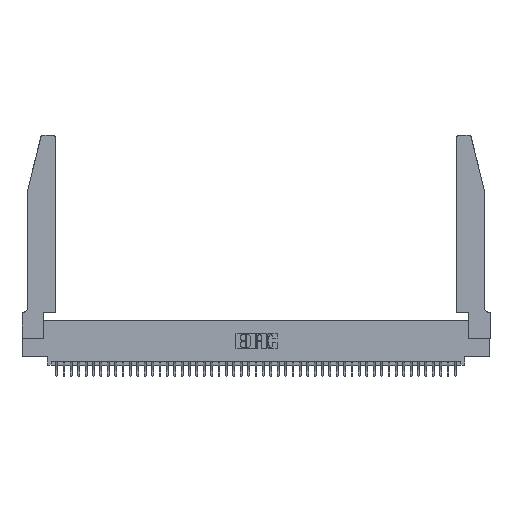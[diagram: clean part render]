
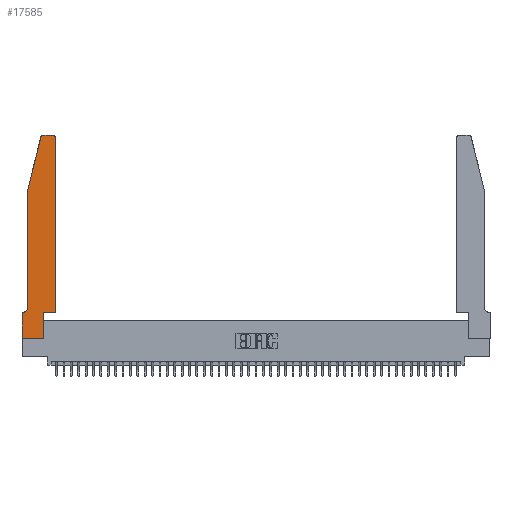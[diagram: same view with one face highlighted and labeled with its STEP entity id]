
A CAD part, top view. The second image highlights one B-rep face of the part: STEP entity #17585.
In plain terms, the highlighted planar face has unit normal (0, 0, 1).
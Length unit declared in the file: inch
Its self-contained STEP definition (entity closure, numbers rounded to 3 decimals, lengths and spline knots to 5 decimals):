
#538 = VECTOR ( 'NONE', #25770, 39.37008 ) ;
#815 = CIRCLE ( 'NONE', #19973, 0.07 ) ;
#1586 = EDGE_CURVE ( 'NONE', #19823, #18015, #17765, .T. ) ;
#2726 = VECTOR ( 'NONE', #23477, 39.37008 ) ;
#3754 = VERTEX_POINT ( 'NONE', #32100 ) ;
#3792 = ORIENTED_EDGE ( 'NONE', *, *, #26870, .T. ) ;
#3825 = AXIS2_PLACEMENT_3D ( 'NONE', #6704, #35289, #6082 ) ;
#4029 = CARTESIAN_POINT ( 'NONE',  ( 0.0755, 2., 0.37 ) ) ;
#4063 = VECTOR ( 'NONE', #32357, 39.37008 ) ;
#4172 = EDGE_CURVE ( 'NONE', #41284, #14350, #6353, .T. ) ;
#4333 = LINE ( 'NONE', #42284, #36367 ) ;
#5212 = AXIS2_PLACEMENT_3D ( 'NONE', #14650, #7881, #11358 ) ;
#6032 = CARTESIAN_POINT ( 'NONE',  ( 0., 0., 0.37 ) ) ;
#6082 = DIRECTION ( 'NONE',  ( 1., 0., 0. ) ) ;
#6353 = LINE ( 'NONE', #34420, #20926 ) ;
#6704 = CARTESIAN_POINT ( 'NONE',  ( 0.4205, 2.72, 0.37 ) ) ;
#7785 = VECTOR ( 'NONE', #24430, 39.37008 ) ;
#7791 = DIRECTION ( 'NONE',  ( -0.239, -0.971, 0. ) ) ;
#7881 = DIRECTION ( 'NONE',  ( 0., 0., 1. ) ) ;
#8245 = DIRECTION ( 'NONE',  ( 0., 0., -1. ) ) ;
#8811 = CARTESIAN_POINT ( 'NONE',  ( 0.2865, 0., 0.37 ) ) ;
#9122 = LINE ( 'NONE', #39452, #4063 ) ;
#11031 = PLANE ( 'NONE',  #5212 ) ;
#11358 = DIRECTION ( 'NONE',  ( 1., 0., 0. ) ) ;
#11810 = ORIENTED_EDGE ( 'NONE', *, *, #4172, .T. ) ;
#12023 = ORIENTED_EDGE ( 'NONE', *, *, #22023, .T. ) ;
#12672 = DIRECTION ( 'NONE',  ( 0., 0., 1. ) ) ;
#13801 = ORIENTED_EDGE ( 'NONE', *, *, #44487, .T. ) ;
#14350 = VERTEX_POINT ( 'NONE', #18992 ) ;
#14650 = CARTESIAN_POINT ( 'NONE',  ( 0., 0.35, 0.37 ) ) ;
#15573 = CARTESIAN_POINT ( 'NONE',  ( 0.4505, 0.35, 0.37 ) ) ;
#15829 = EDGE_LOOP ( 'NONE', ( #20323, #28314, #13801, #29531, #16729, #11810, #28741, #21027, #28613, #3792, #32587, #12023 ) ) ;
#15952 = CARTESIAN_POINT ( 'NONE',  ( 0.4505, 0.35, 0.37 ) ) ;
#16729 = ORIENTED_EDGE ( 'NONE', *, *, #18944, .T. ) ;
#16862 = CIRCLE ( 'NONE', #3825, 0.03 ) ;
#17291 = CARTESIAN_POINT ( 'NONE',  ( 0.25487, 2.72718, 0.37 ) ) ;
#17585 = ADVANCED_FACE ( 'NONE', ( #38075 ), #11031, .T. ) ;
#17765 = CIRCLE ( 'NONE', #27639, 0.03 ) ;
#18015 = VERTEX_POINT ( 'NONE', #17291 ) ;
#18274 = CARTESIAN_POINT ( 'NONE',  ( 0., 0., 0.37 ) ) ;
#18944 = EDGE_CURVE ( 'NONE', #3754, #41284, #815, .T. ) ;
#18992 = CARTESIAN_POINT ( 'NONE',  ( 0., 0.35, 0.37 ) ) ;
#19054 = DIRECTION ( 'NONE',  ( -1., 0., 0. ) ) ;
#19436 = CARTESIAN_POINT ( 'NONE',  ( 0.0055, 0.35, 0.37 ) ) ;
#19531 = DIRECTION ( 'NONE',  ( 1., 0., 0. ) ) ;
#19630 = VERTEX_POINT ( 'NONE', #8811 ) ;
#19657 = CARTESIAN_POINT ( 'NONE',  ( 0.2865, 0.35, 0.37 ) ) ;
#19823 = VERTEX_POINT ( 'NONE', #23278 ) ;
#19973 = AXIS2_PLACEMENT_3D ( 'NONE', #22684, #8245, #19054 ) ;
#20323 = ORIENTED_EDGE ( 'NONE', *, *, #27969, .T. ) ;
#20500 = CARTESIAN_POINT ( 'NONE',  ( 0.4505, 2.72, 0.37 ) ) ;
#20820 = CARTESIAN_POINT ( 'NONE',  ( 0.2605, 2.75, 0.37 ) ) ;
#20921 = DIRECTION ( 'NONE',  ( 1., 0., 0. ) ) ;
#20926 = VECTOR ( 'NONE', #25094, 39.37008 ) ;
#21027 = ORIENTED_EDGE ( 'NONE', *, *, #28450, .T. ) ;
#21094 = EDGE_CURVE ( 'NONE', #35872, #3754, #43291, .T. ) ;
#21793 = LINE ( 'NONE', #19657, #2726 ) ;
#22023 = EDGE_CURVE ( 'NONE', #27707, #37487, #16862, .T. ) ;
#22375 = VECTOR ( 'NONE', #20921, 39.37008 ) ;
#22684 = CARTESIAN_POINT ( 'NONE',  ( 0.0055, 0.42, 0.37 ) ) ;
#23278 = CARTESIAN_POINT ( 'NONE',  ( 0.284, 2.75, 0.37 ) ) ;
#23477 = DIRECTION ( 'NONE',  ( 0., 1., 0. ) ) ;
#24430 = DIRECTION ( 'NONE',  ( -1., 0., 0. ) ) ;
#25094 = DIRECTION ( 'NONE',  ( -1., 0., 0. ) ) ;
#25174 = CARTESIAN_POINT ( 'NONE',  ( 0.0755, 2., 0.37 ) ) ;
#25770 = DIRECTION ( 'NONE',  ( 0., -1., 0. ) ) ;
#26344 = LINE ( 'NONE', #20820, #7785 ) ;
#26870 = EDGE_CURVE ( 'NONE', #32142, #33452, #44471, .T. ) ;
#27639 = AXIS2_PLACEMENT_3D ( 'NONE', #30398, #12672, #19531 ) ;
#27707 = VERTEX_POINT ( 'NONE', #20500 ) ;
#27968 = DIRECTION ( 'NONE',  ( 0., 1., 0. ) ) ;
#27969 = EDGE_CURVE ( 'NONE', #37487, #19823, #26344, .T. ) ;
#28314 = ORIENTED_EDGE ( 'NONE', *, *, #1586, .T. ) ;
#28450 = EDGE_CURVE ( 'NONE', #32233, #19630, #38135, .T. ) ;
#28613 = ORIENTED_EDGE ( 'NONE', *, *, #38099, .T. ) ;
#28741 = ORIENTED_EDGE ( 'NONE', *, *, #34393, .T. ) ;
#29072 = LINE ( 'NONE', #4029, #35833 ) ;
#29531 = ORIENTED_EDGE ( 'NONE', *, *, #21094, .T. ) ;
#29675 = CARTESIAN_POINT ( 'NONE',  ( 0.0755, 2., 0.37 ) ) ;
#30398 = CARTESIAN_POINT ( 'NONE',  ( 0.284, 2.72, 0.37 ) ) ;
#31551 = EDGE_CURVE ( 'NONE', #33452, #27707, #4333, .T. ) ;
#32100 = CARTESIAN_POINT ( 'NONE',  ( 0.0755, 0.42, 0.37 ) ) ;
#32142 = VERTEX_POINT ( 'NONE', #32897 ) ;
#32233 = VERTEX_POINT ( 'NONE', #18274 ) ;
#32357 = DIRECTION ( 'NONE',  ( 0., -1., 0. ) ) ;
#32587 = ORIENTED_EDGE ( 'NONE', *, *, #31551, .T. ) ;
#32897 = CARTESIAN_POINT ( 'NONE',  ( 0.2865, 0.35, 0.37 ) ) ;
#33452 = VERTEX_POINT ( 'NONE', #15952 ) ;
#34393 = EDGE_CURVE ( 'NONE', #14350, #32233, #9122, .T. ) ;
#34420 = CARTESIAN_POINT ( 'NONE',  ( 0.0755, 0.35, 0.37 ) ) ;
#35289 = DIRECTION ( 'NONE',  ( 0., 0., 1. ) ) ;
#35833 = VECTOR ( 'NONE', #7791, 39.37008 ) ;
#35872 = VERTEX_POINT ( 'NONE', #25174 ) ;
#36367 = VECTOR ( 'NONE', #27968, 39.37008 ) ;
#37487 = VERTEX_POINT ( 'NONE', #45820 ) ;
#38075 = FACE_OUTER_BOUND ( 'NONE', #15829, .T. ) ;
#38099 = EDGE_CURVE ( 'NONE', #19630, #32142, #21793, .T. ) ;
#38135 = LINE ( 'NONE', #6032, #22375 ) ;
#39452 = CARTESIAN_POINT ( 'NONE',  ( 0., 0., 0.37 ) ) ;
#41284 = VERTEX_POINT ( 'NONE', #19436 ) ;
#42284 = CARTESIAN_POINT ( 'NONE',  ( 0.4505, 0.35, 0.37 ) ) ;
#43291 = LINE ( 'NONE', #29675, #538 ) ;
#43327 = VECTOR ( 'NONE', #44467, 39.37008 ) ;
#44467 = DIRECTION ( 'NONE',  ( 1., 0., 0. ) ) ;
#44471 = LINE ( 'NONE', #15573, #43327 ) ;
#44487 = EDGE_CURVE ( 'NONE', #18015, #35872, #29072, .T. ) ;
#45820 = CARTESIAN_POINT ( 'NONE',  ( 0.4205, 2.75, 0.37 ) ) ;
